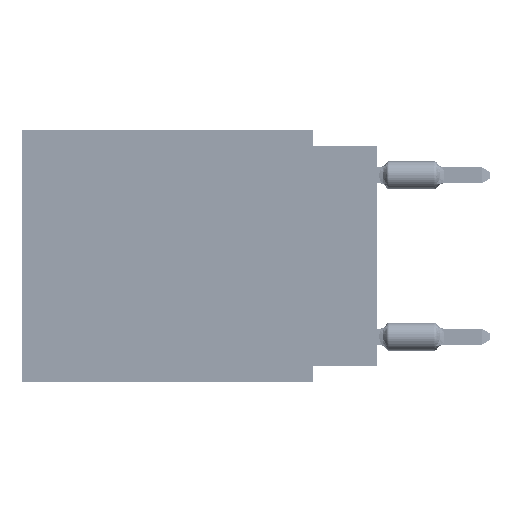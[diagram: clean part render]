
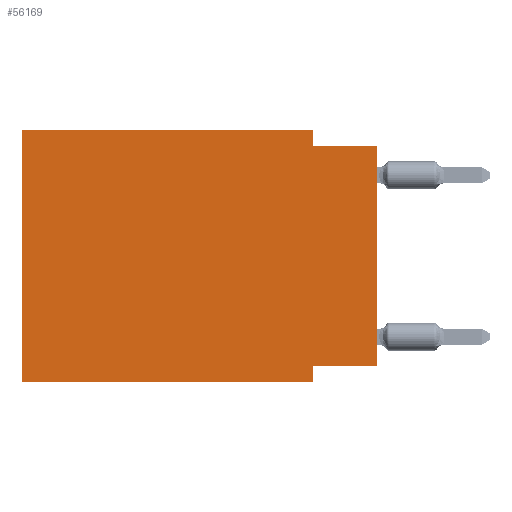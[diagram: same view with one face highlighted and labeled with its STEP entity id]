
A CAD part, left-side view. The second image highlights one B-rep face of the part: STEP entity #56169.
In plain terms, the highlighted planar face has unit normal (-1, 0, 0).
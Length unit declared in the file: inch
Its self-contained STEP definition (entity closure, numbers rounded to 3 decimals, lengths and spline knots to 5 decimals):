
#53 = DIRECTION ( 'NONE',  ( 0., 0., -1. ) ) ;
#3914 = LINE ( 'NONE', #10554, #18333 ) ;
#4031 = EDGE_CURVE ( 'NONE', #18362, #6480, #68456, .T. ) ;
#5137 = CARTESIAN_POINT ( 'NONE',  ( 0., 0.1, 0. ) ) ;
#6480 = VERTEX_POINT ( 'NONE', #46889 ) ;
#6679 = FACE_OUTER_BOUND ( 'NONE', #57218, .T. ) ;
#6853 = ORIENTED_EDGE ( 'NONE', *, *, #48028, .F. ) ;
#7090 = LINE ( 'NONE', #54888, #54106 ) ;
#7349 = VERTEX_POINT ( 'NONE', #9914 ) ;
#8358 = VECTOR ( 'NONE', #18004, 39.37008 ) ;
#8558 = CARTESIAN_POINT ( 'NONE',  ( 0., 0., -0.365 ) ) ;
#9321 = LINE ( 'NONE', #8558, #67542 ) ;
#9579 = ORIENTED_EDGE ( 'NONE', *, *, #4031, .T. ) ;
#9705 = DIRECTION ( 'NONE',  ( 0., 0., 1. ) ) ;
#9734 = EDGE_CURVE ( 'NONE', #50924, #28546, #7090, .T. ) ;
#9914 = CARTESIAN_POINT ( 'NONE',  ( 0., 0.55, 0. ) ) ;
#10554 = CARTESIAN_POINT ( 'NONE',  ( 0., 0.55, 0. ) ) ;
#10622 = VECTOR ( 'NONE', #21026, 39.37008 ) ;
#15257 = CARTESIAN_POINT ( 'NONE',  ( 0., 0.55, 0. ) ) ;
#16893 = EDGE_CURVE ( 'NONE', #62104, #28546, #58797, .T. ) ;
#17227 = EDGE_CURVE ( 'NONE', #18362, #7349, #74047, .T. ) ;
#18004 = DIRECTION ( 'NONE',  ( 0., -1., 0. ) ) ;
#18333 = VECTOR ( 'NONE', #45444, 39.37008 ) ;
#18362 = VERTEX_POINT ( 'NONE', #66655 ) ;
#18454 = EDGE_CURVE ( 'NONE', #7349, #36032, #3914, .T. ) ;
#21026 = DIRECTION ( 'NONE',  ( 0., -1., 0. ) ) ;
#22761 = DIRECTION ( 'NONE',  ( 0., 0., -1. ) ) ;
#22977 = CARTESIAN_POINT ( 'NONE',  ( 0., 0.1, 0. ) ) ;
#23774 = VECTOR ( 'NONE', #22761, 39.37008 ) ;
#24700 = PLANE ( 'NONE',  #28472 ) ;
#26335 = EDGE_CURVE ( 'NONE', #36032, #62104, #34925, .T. ) ;
#28472 = AXIS2_PLACEMENT_3D ( 'NONE', #48583, #37224, #66619 ) ;
#28546 = VERTEX_POINT ( 'NONE', #56278 ) ;
#32453 = DIRECTION ( 'NONE',  ( 0., 1., 0. ) ) ;
#34925 = LINE ( 'NONE', #5137, #48439 ) ;
#36032 = VERTEX_POINT ( 'NONE', #22977 ) ;
#37018 = ORIENTED_EDGE ( 'NONE', *, *, #17227, .F. ) ;
#37224 = DIRECTION ( 'NONE',  ( 1., 0., 0. ) ) ;
#37363 = VERTEX_POINT ( 'NONE', #60171 ) ;
#38408 = ORIENTED_EDGE ( 'NONE', *, *, #18454, .F. ) ;
#44692 = VECTOR ( 'NONE', #50893, 39.37008 ) ;
#45306 = ORIENTED_EDGE ( 'NONE', *, *, #16893, .F. ) ;
#45444 = DIRECTION ( 'NONE',  ( 0., -1., 0. ) ) ;
#46266 = LINE ( 'NONE', #47033, #23774 ) ;
#46620 = CARTESIAN_POINT ( 'NONE',  ( 0., 0.1, -0.025 ) ) ;
#46889 = CARTESIAN_POINT ( 'NONE',  ( 0., 0.1, -0.39 ) ) ;
#47033 = CARTESIAN_POINT ( 'NONE',  ( 0., 0.1, -0.39 ) ) ;
#47787 = CARTESIAN_POINT ( 'NONE',  ( 0., 0., -0.025 ) ) ;
#48028 = EDGE_CURVE ( 'NONE', #37363, #6480, #46266, .T. ) ;
#48439 = VECTOR ( 'NONE', #53, 39.37008 ) ;
#48583 = CARTESIAN_POINT ( 'NONE',  ( 0., 0.55, 0. ) ) ;
#50893 = DIRECTION ( 'NONE',  ( 0., 0., 1. ) ) ;
#50924 = VERTEX_POINT ( 'NONE', #61412 ) ;
#54106 = VECTOR ( 'NONE', #9705, 39.37008 ) ;
#54888 = CARTESIAN_POINT ( 'NONE',  ( 0., 0., 0. ) ) ;
#56169 = ADVANCED_FACE ( 'NONE', ( #6679 ), #24700, .F. ) ;
#56278 = CARTESIAN_POINT ( 'NONE',  ( 0., 0., -0.025 ) ) ;
#57218 = EDGE_LOOP ( 'NONE', ( #64254, #45306, #66982, #38408, #37018, #9579, #6853, #72311 ) ) ;
#58797 = LINE ( 'NONE', #47787, #8358 ) ;
#60171 = CARTESIAN_POINT ( 'NONE',  ( 0., 0.1, -0.365 ) ) ;
#61412 = CARTESIAN_POINT ( 'NONE',  ( 0., 0., -0.365 ) ) ;
#62104 = VERTEX_POINT ( 'NONE', #46620 ) ;
#64254 = ORIENTED_EDGE ( 'NONE', *, *, #9734, .T. ) ;
#66619 = DIRECTION ( 'NONE',  ( 0., 0., -1. ) ) ;
#66655 = CARTESIAN_POINT ( 'NONE',  ( 0., 0.55, -0.39 ) ) ;
#66982 = ORIENTED_EDGE ( 'NONE', *, *, #26335, .F. ) ;
#67542 = VECTOR ( 'NONE', #32453, 39.37008 ) ;
#68456 = LINE ( 'NONE', #73166, #10622 ) ;
#72311 = ORIENTED_EDGE ( 'NONE', *, *, #75011, .F. ) ;
#73166 = CARTESIAN_POINT ( 'NONE',  ( 0., 0.55, -0.39 ) ) ;
#74047 = LINE ( 'NONE', #15257, #44692 ) ;
#75011 = EDGE_CURVE ( 'NONE', #50924, #37363, #9321, .T. ) ;
